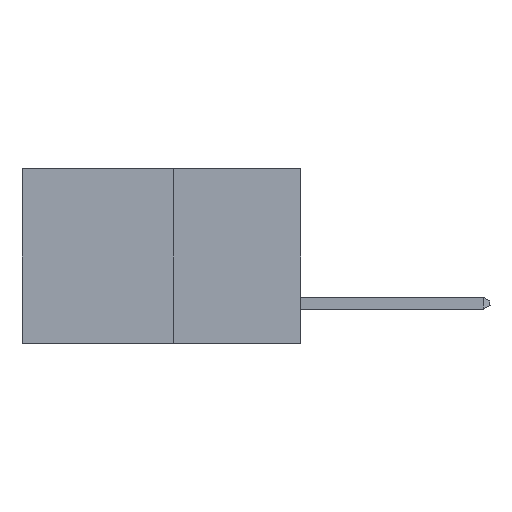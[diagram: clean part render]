
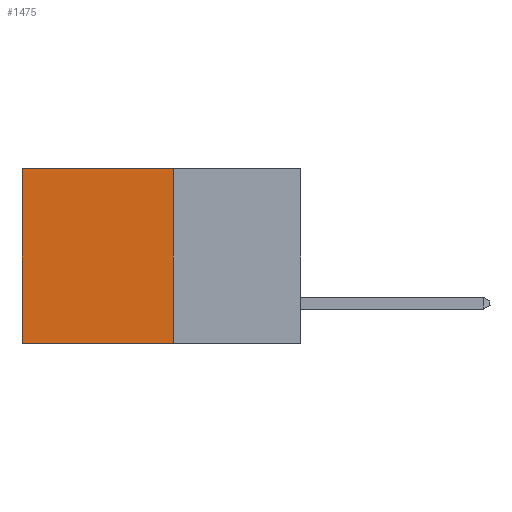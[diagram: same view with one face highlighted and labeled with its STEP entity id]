
A CAD part, left-side view. The second image highlights one B-rep face of the part: STEP entity #1475.
In plain terms, the highlighted planar face has unit normal (-1, 0, 0).
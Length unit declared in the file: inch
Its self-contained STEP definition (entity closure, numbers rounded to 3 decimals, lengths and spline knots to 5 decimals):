
#80 = LINE ( 'NONE', #18123, #17619 ) ;
#140 = LINE ( 'NONE', #18029, #11311 ) ;
#444 = LINE ( 'NONE', #13061, #11587 ) ;
#986 = VERTEX_POINT ( 'NONE', #12610 ) ;
#1093 = DIRECTION ( 'NONE',  ( 0., 0., -1. ) ) ;
#1475 = ADVANCED_FACE ( 'NONE', ( #10840 ), #13509, .F. ) ;
#1756 = EDGE_LOOP ( 'NONE', ( #16218, #9834, #14352, #16459 ) ) ;
#1979 = CARTESIAN_POINT ( 'NONE',  ( 0.277, 0.59, -0.37 ) ) ;
#2783 = CARTESIAN_POINT ( 'NONE',  ( 0.277, 0.27, -0.37 ) ) ;
#3704 = EDGE_CURVE ( 'NONE', #8450, #5956, #444, .T. ) ;
#5428 = LINE ( 'NONE', #12656, #5891 ) ;
#5520 = DIRECTION ( 'NONE',  ( 0., 0., -1. ) ) ;
#5891 = VECTOR ( 'NONE', #12488, 39.37008 ) ;
#5956 = VERTEX_POINT ( 'NONE', #1979 ) ;
#7287 = CARTESIAN_POINT ( 'NONE',  ( 0.277, 0.59, 0. ) ) ;
#8450 = VERTEX_POINT ( 'NONE', #7287 ) ;
#8812 = EDGE_CURVE ( 'NONE', #10660, #5956, #80, .T. ) ;
#9532 = EDGE_CURVE ( 'NONE', #986, #8450, #5428, .T. ) ;
#9834 = ORIENTED_EDGE ( 'NONE', *, *, #8812, .F. ) ;
#10660 = VERTEX_POINT ( 'NONE', #2783 ) ;
#10840 = FACE_OUTER_BOUND ( 'NONE', #1756, .T. ) ;
#11158 = AXIS2_PLACEMENT_3D ( 'NONE', #12650, #17917, #13218 ) ;
#11311 = VECTOR ( 'NONE', #1093, 39.37008 ) ;
#11587 = VECTOR ( 'NONE', #5520, 39.37008 ) ;
#12488 = DIRECTION ( 'NONE',  ( 0., 1., 0. ) ) ;
#12610 = CARTESIAN_POINT ( 'NONE',  ( 0.277, 0.27, 0. ) ) ;
#12650 = CARTESIAN_POINT ( 'NONE',  ( 0.277, 0.27, -0.37 ) ) ;
#12656 = CARTESIAN_POINT ( 'NONE',  ( 0.277, 0.27, 0. ) ) ;
#13061 = CARTESIAN_POINT ( 'NONE',  ( 0.277, 0.59, -0.37 ) ) ;
#13218 = DIRECTION ( 'NONE',  ( 0., 0., -1. ) ) ;
#13287 = EDGE_CURVE ( 'NONE', #986, #10660, #140, .T. ) ;
#13509 = PLANE ( 'NONE',  #11158 ) ;
#14352 = ORIENTED_EDGE ( 'NONE', *, *, #13287, .F. ) ;
#16218 = ORIENTED_EDGE ( 'NONE', *, *, #3704, .T. ) ;
#16459 = ORIENTED_EDGE ( 'NONE', *, *, #9532, .T. ) ;
#17619 = VECTOR ( 'NONE', #18233, 39.37008 ) ;
#17917 = DIRECTION ( 'NONE',  ( 1., 0., 0. ) ) ;
#18029 = CARTESIAN_POINT ( 'NONE',  ( 0.277, 0.27, -0.37 ) ) ;
#18123 = CARTESIAN_POINT ( 'NONE',  ( 0.277, 0.27, -0.37 ) ) ;
#18233 = DIRECTION ( 'NONE',  ( 0., 1., 0. ) ) ;
